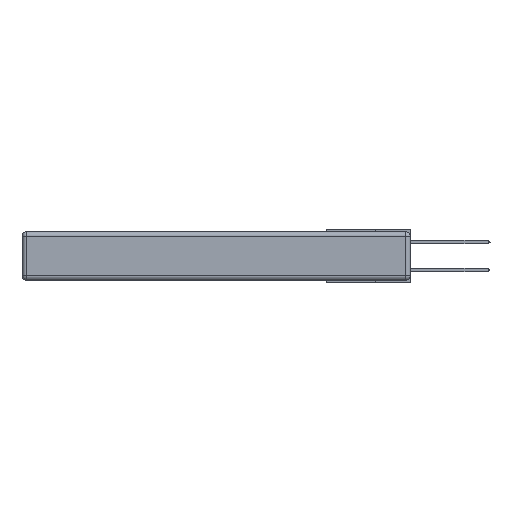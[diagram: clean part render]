
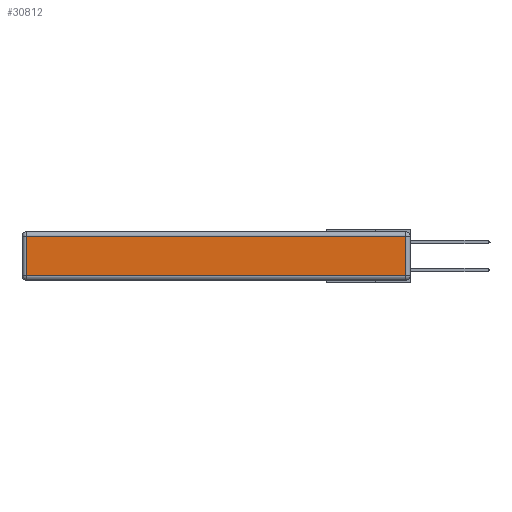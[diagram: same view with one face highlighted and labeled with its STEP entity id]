
A CAD part, left-side view. The second image highlights one B-rep face of the part: STEP entity #30812.
In plain terms, the highlighted planar face has unit normal (-1, 0, 0).
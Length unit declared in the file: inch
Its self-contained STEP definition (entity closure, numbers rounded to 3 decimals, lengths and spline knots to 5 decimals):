
#1465 = PLANE ( 'NONE',  #5215 ) ;
#3389 = CARTESIAN_POINT ( 'NONE',  ( 0., 2.72, -0.313 ) ) ;
#3740 = CARTESIAN_POINT ( 'NONE',  ( 0., 0., -0.313 ) ) ;
#4662 = DIRECTION ( 'NONE',  ( 0., 0., 1. ) ) ;
#5130 = LINE ( 'NONE', #27934, #31068 ) ;
#5215 = AXIS2_PLACEMENT_3D ( 'NONE', #19535, #19871, #25197 ) ;
#5631 = VECTOR ( 'NONE', #25602, 39.37008 ) ;
#6092 = EDGE_LOOP ( 'NONE', ( #30076, #6585, #12618, #9539 ) ) ;
#6585 = ORIENTED_EDGE ( 'NONE', *, *, #10303, .T. ) ;
#6966 = EDGE_CURVE ( 'NONE', #14848, #23646, #26643, .T. ) ;
#8153 = FACE_OUTER_BOUND ( 'NONE', #6092, .T. ) ;
#8695 = CARTESIAN_POINT ( 'NONE',  ( 0., 0.03, -0.313 ) ) ;
#8938 = DIRECTION ( 'NONE',  ( 0., -1., 0. ) ) ;
#9539 = ORIENTED_EDGE ( 'NONE', *, *, #6966, .T. ) ;
#10303 = EDGE_CURVE ( 'NONE', #19267, #26435, #12105, .T. ) ;
#12105 = LINE ( 'NONE', #24838, #32228 ) ;
#12618 = ORIENTED_EDGE ( 'NONE', *, *, #26746, .T. ) ;
#13728 = CARTESIAN_POINT ( 'NONE',  ( 0., 2.72, -0.03 ) ) ;
#14848 = VERTEX_POINT ( 'NONE', #13728 ) ;
#17457 = DIRECTION ( 'NONE',  ( 0., 1., 0. ) ) ;
#17985 = CARTESIAN_POINT ( 'NONE',  ( 0., 2.72, -0.343 ) ) ;
#19267 = VERTEX_POINT ( 'NONE', #8695 ) ;
#19535 = CARTESIAN_POINT ( 'NONE',  ( 0., 0., -0.343 ) ) ;
#19871 = DIRECTION ( 'NONE',  ( -1., 0., 0. ) ) ;
#23646 = VERTEX_POINT ( 'NONE', #3389 ) ;
#24523 = CARTESIAN_POINT ( 'NONE',  ( 0., 0.03, -0.03 ) ) ;
#24598 = VECTOR ( 'NONE', #8938, 39.37008 ) ;
#24838 = CARTESIAN_POINT ( 'NONE',  ( 0., 0.03, -0.343 ) ) ;
#25197 = DIRECTION ( 'NONE',  ( 0., 0., 1. ) ) ;
#25602 = DIRECTION ( 'NONE',  ( 0., 0., -1. ) ) ;
#26031 = EDGE_CURVE ( 'NONE', #23646, #19267, #33205, .T. ) ;
#26435 = VERTEX_POINT ( 'NONE', #24523 ) ;
#26643 = LINE ( 'NONE', #17985, #5631 ) ;
#26746 = EDGE_CURVE ( 'NONE', #26435, #14848, #5130, .T. ) ;
#27934 = CARTESIAN_POINT ( 'NONE',  ( 0., 2.75, -0.03 ) ) ;
#30076 = ORIENTED_EDGE ( 'NONE', *, *, #26031, .T. ) ;
#30812 = ADVANCED_FACE ( 'NONE', ( #8153 ), #1465, .T. ) ;
#31068 = VECTOR ( 'NONE', #17457, 39.37008 ) ;
#32228 = VECTOR ( 'NONE', #4662, 39.37008 ) ;
#33205 = LINE ( 'NONE', #3740, #24598 ) ;
